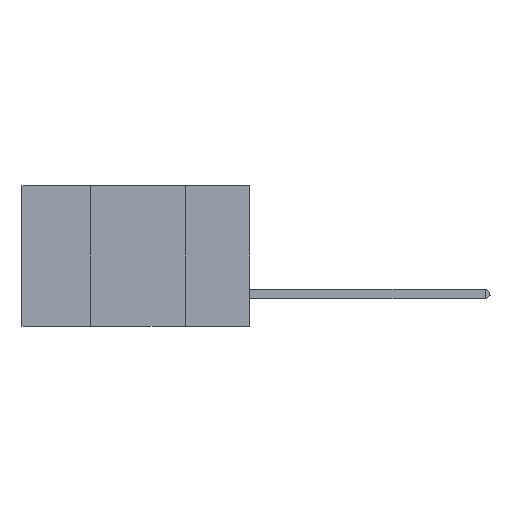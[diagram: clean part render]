
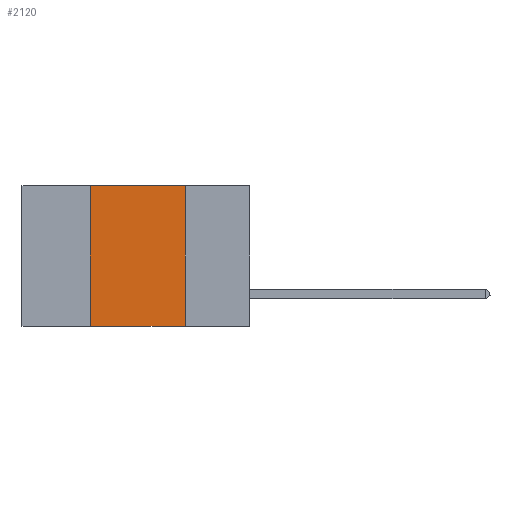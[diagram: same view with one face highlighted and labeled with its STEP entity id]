
A CAD part, left-side view. The second image highlights one B-rep face of the part: STEP entity #2120.
In plain terms, the highlighted planar face has unit normal (-1, 0, 0).
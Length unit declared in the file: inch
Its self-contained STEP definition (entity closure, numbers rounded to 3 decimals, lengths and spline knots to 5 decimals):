
#224 = EDGE_CURVE ( 'NONE', #4625, #1399, #660, .T. ) ;
#471 = EDGE_CURVE ( 'NONE', #10980, #4625, #8053, .T. ) ;
#660 = LINE ( 'NONE', #7342, #11256 ) ;
#714 = ORIENTED_EDGE ( 'NONE', *, *, #11544, .F. ) ;
#864 = ORIENTED_EDGE ( 'NONE', *, *, #471, .F. ) ;
#1122 = CARTESIAN_POINT ( 'NONE',  ( 0., 0.6, 0. ) ) ;
#1399 = VERTEX_POINT ( 'NONE', #4979 ) ;
#1681 = LINE ( 'NONE', #10379, #9392 ) ;
#1965 = CARTESIAN_POINT ( 'NONE',  ( 0., 0.17, -0.37 ) ) ;
#2120 = ADVANCED_FACE ( 'NONE', ( #3589 ), #9563, .F. ) ;
#3589 = FACE_OUTER_BOUND ( 'NONE', #8114, .T. ) ;
#3725 = AXIS2_PLACEMENT_3D ( 'NONE', #1122, #9481, #4910 ) ;
#3969 = CARTESIAN_POINT ( 'NONE',  ( 0., 0.42, 0. ) ) ;
#4114 = ORIENTED_EDGE ( 'NONE', *, *, #5481, .T. ) ;
#4625 = VERTEX_POINT ( 'NONE', #8939 ) ;
#4787 = DIRECTION ( 'NONE',  ( 0., 0., -1. ) ) ;
#4910 = DIRECTION ( 'NONE',  ( 0., 0., -1. ) ) ;
#4979 = CARTESIAN_POINT ( 'NONE',  ( 0., 0.17, 0. ) ) ;
#5481 = EDGE_CURVE ( 'NONE', #10980, #11475, #6996, .T. ) ;
#5715 = VECTOR ( 'NONE', #11511, 39.37008 ) ;
#6996 = LINE ( 'NONE', #8717, #5715 ) ;
#7342 = CARTESIAN_POINT ( 'NONE',  ( 0., 0.6, 0. ) ) ;
#8053 = LINE ( 'NONE', #3969, #9944 ) ;
#8114 = EDGE_LOOP ( 'NONE', ( #714, #9523, #864, #4114 ) ) ;
#8256 = DIRECTION ( 'NONE',  ( 0., -1., 0. ) ) ;
#8717 = CARTESIAN_POINT ( 'NONE',  ( 0., 0.6, -0.37 ) ) ;
#8768 = CARTESIAN_POINT ( 'NONE',  ( 0., 0.42, -0.37 ) ) ;
#8939 = CARTESIAN_POINT ( 'NONE',  ( 0., 0.42, 0. ) ) ;
#9392 = VECTOR ( 'NONE', #4787, 39.37008 ) ;
#9481 = DIRECTION ( 'NONE',  ( 1., 0., 0. ) ) ;
#9523 = ORIENTED_EDGE ( 'NONE', *, *, #224, .F. ) ;
#9563 = PLANE ( 'NONE',  #3725 ) ;
#9633 = DIRECTION ( 'NONE',  ( 0., 0., 1. ) ) ;
#9944 = VECTOR ( 'NONE', #9633, 39.37008 ) ;
#10379 = CARTESIAN_POINT ( 'NONE',  ( 0., 0.17, 0. ) ) ;
#10980 = VERTEX_POINT ( 'NONE', #8768 ) ;
#11256 = VECTOR ( 'NONE', #8256, 39.37008 ) ;
#11475 = VERTEX_POINT ( 'NONE', #1965 ) ;
#11511 = DIRECTION ( 'NONE',  ( 0., -1., 0. ) ) ;
#11544 = EDGE_CURVE ( 'NONE', #1399, #11475, #1681, .T. ) ;
